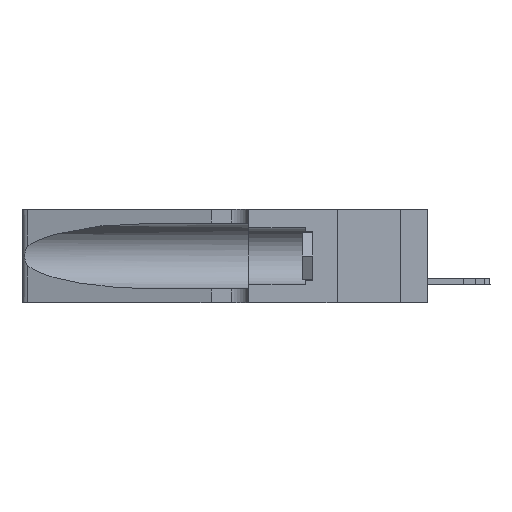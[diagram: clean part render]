
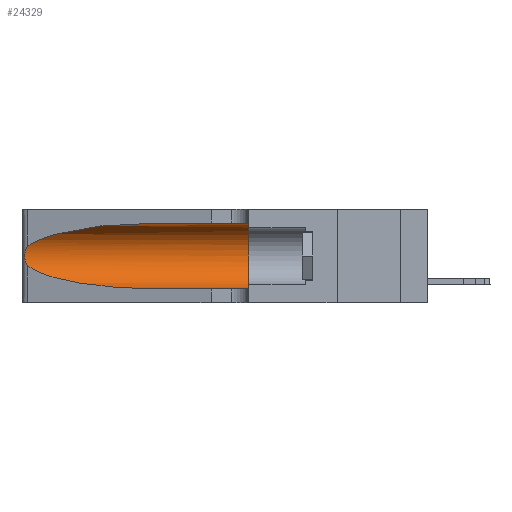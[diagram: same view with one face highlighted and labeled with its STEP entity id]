
A CAD part, left-side view. The second image highlights one B-rep face of the part: STEP entity #24329.
In plain terms, the highlighted cylindrical face has radius 3.308 mm (diameter 6.617 mm), a partial arc.
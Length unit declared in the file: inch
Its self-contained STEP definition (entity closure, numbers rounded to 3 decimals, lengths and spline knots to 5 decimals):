
#185 = VERTEX_POINT ( 'NONE', #25249 ) ;
#747 = ORIENTED_EDGE ( 'NONE', *, *, #14140, .T. ) ;
#1238 = CARTESIAN_POINT ( 'NONE',  ( 0.25487, 1.22718, 0.14631 ) ) ;
#2721 = CARTESIAN_POINT ( 'NONE',  ( 0.1305, 0.35, 0.31525 ) ) ;
#3000 = EDGE_CURVE ( 'NONE', #185, #18550, #15480, .T. ) ;
#3093 = CARTESIAN_POINT ( 'NONE',  ( 0.2373, 1.15595, 0.08982 ) ) ;
#3687 = EDGE_CURVE ( 'NONE', #185, #5527, #24208, .T. ) ;
#4220 = VERTEX_POINT ( 'NONE', #15285 ) ;
#4230 = CARTESIAN_POINT ( 'NONE',  ( 0.25487, 1.22718, 0.22369 ) ) ;
#4458 = CARTESIAN_POINT ( 'NONE',  ( 0.18966, 0.96281, 0.05475 ) ) ;
#4460 = CARTESIAN_POINT ( 'NONE',  ( 0.18966, 0.96281, 0.31525 ) ) ;
#4699 = ORIENTED_EDGE ( 'NONE', *, *, #13871, .T. ) ;
#5527 = VERTEX_POINT ( 'NONE', #9774 ) ;
#6185 = CARTESIAN_POINT ( 'NONE',  ( 0.25854, 1.2359, 0.20912 ) ) ;
#6305 = ORIENTED_EDGE ( 'NONE', *, *, #18896, .F. ) ;
#6319 = CARTESIAN_POINT ( 'NONE',  ( 0.1305, 0.72297, 0.31525 ) ) ;
#7128 = CARTESIAN_POINT ( 'NONE',  ( 0.25856, 1.23593, 0.16098 ) ) ;
#7228 = CARTESIAN_POINT ( 'NONE',  ( 0.25555, 1.22993, 0.14849 ) ) ;
#7884 = VECTOR ( 'NONE', #17106, 39.37008 ) ;
#8335 = CARTESIAN_POINT ( 'NONE',  ( 0.26075, 1.23896, 0.19203 ) ) ;
#8352 = AXIS2_PLACEMENT_3D ( 'NONE', #9111, #23697, #17482 ) ;
#8457 = CARTESIAN_POINT ( 'NONE',  ( 0.1305, 1.61858, 0.185 ) ) ;
#9111 = CARTESIAN_POINT ( 'NONE',  ( 0.1305, 0.35, 0.185 ) ) ;
#9644 = FACE_OUTER_BOUND ( 'NONE', #22752, .T. ) ;
#9720 = DIRECTION ( 'NONE',  ( 0., -1., 0. ) ) ;
#9774 = CARTESIAN_POINT ( 'NONE',  ( 0.25487, 1.22718, 0.22369 ) ) ;
#10078 = ORIENTED_EDGE ( 'NONE', *, *, #15621, .T. ) ;
#10710 =( BOUNDED_CURVE ( )  B_SPLINE_CURVE ( 3, ( #12504, #3093, #4458, #14472 ),
 .UNSPECIFIED., .F., .T. ) 
 B_SPLINE_CURVE_WITH_KNOTS ( ( 4, 4 ),
 ( 3.44316, 4.71239 ),
 .UNSPECIFIED. ) 
 CURVE ( )  GEOMETRIC_REPRESENTATION_ITEM ( )  RATIONAL_B_SPLINE_CURVE ( ( 1., 0.87, 0.87, 1. ) ) 
 REPRESENTATION_ITEM ( '' )  );
#11122 = AXIS2_PLACEMENT_3D ( 'NONE', #8457, #24713, #12396 ) ;
#12005 = CARTESIAN_POINT ( 'NONE',  ( 0.1305, 1.61858, 0.05475 ) ) ;
#12299 = CIRCLE ( 'NONE', #8352, 0.13025 ) ;
#12396 = DIRECTION ( 'NONE',  ( 0., 0., -1. ) ) ;
#12504 = CARTESIAN_POINT ( 'NONE',  ( 0.25487, 1.22718, 0.14631 ) ) ;
#13797 = VERTEX_POINT ( 'NONE', #20514 ) ;
#13871 = EDGE_CURVE ( 'NONE', #24351, #13797, #10710, .T. ) ;
#14140 = EDGE_CURVE ( 'NONE', #5527, #24351, #18557, .T. ) ;
#14472 = CARTESIAN_POINT ( 'NONE',  ( 0.1305, 0.72297, 0.05475 ) ) ;
#14692 = CYLINDRICAL_SURFACE ( 'NONE', #11122, 0.13025 ) ;
#15026 = CARTESIAN_POINT ( 'NONE',  ( 0.25789, 1.23486, 0.15765 ) ) ;
#15285 = CARTESIAN_POINT ( 'NONE',  ( 0.1305, 0.35, 0.05475 ) ) ;
#15480 = LINE ( 'NONE', #24943, #7884 ) ;
#15621 = EDGE_CURVE ( 'NONE', #13797, #4220, #15828, .T. ) ;
#15828 = LINE ( 'NONE', #12005, #22567 ) ;
#16533 = CARTESIAN_POINT ( 'NONE',  ( 0.2373, 1.15595, 0.28018 ) ) ;
#17106 = DIRECTION ( 'NONE',  ( 0., -1., 0. ) ) ;
#17187 = CARTESIAN_POINT ( 'NONE',  ( 0.26017, 1.23833, 0.17102 ) ) ;
#17482 = DIRECTION ( 'NONE',  ( 0., 0., 1. ) ) ;
#18550 = VERTEX_POINT ( 'NONE', #2721 ) ;
#18557 = B_SPLINE_CURVE_WITH_KNOTS ( 'NONE', 3,
 ( #4230, #22617, #24765, #20546, #6185, #20468, #8335, #18648, #17187, #7128, #15026, #23482, #7228, #1238 ),
 .UNSPECIFIED., .F., .F.,
 ( 4, 2, 2, 2, 2, 2, 4 ),
 ( 0., 0.00027, 0.00053, 0.00107, 0.0016, 0.00187, 0.00214 ),
 .UNSPECIFIED. ) ;
#18648 = CARTESIAN_POINT ( 'NONE',  ( 0.26075, 1.23896, 0.178 ) ) ;
#18896 = EDGE_CURVE ( 'NONE', #18550, #4220, #12299, .T. ) ;
#20468 = CARTESIAN_POINT ( 'NONE',  ( 0.26018, 1.23835, 0.19895 ) ) ;
#20514 = CARTESIAN_POINT ( 'NONE',  ( 0.1305, 0.72297, 0.05475 ) ) ;
#20546 = CARTESIAN_POINT ( 'NONE',  ( 0.25787, 1.23484, 0.2124 ) ) ;
#22567 = VECTOR ( 'NONE', #9720, 39.37008 ) ;
#22617 = CARTESIAN_POINT ( 'NONE',  ( 0.25555, 1.22994, 0.2215 ) ) ;
#22674 = CARTESIAN_POINT ( 'NONE',  ( 0.25487, 1.22718, 0.22369 ) ) ;
#22752 = EDGE_LOOP ( 'NONE', ( #23174, #747, #4699, #10078, #6305, #22986 ) ) ;
#22986 = ORIENTED_EDGE ( 'NONE', *, *, #3000, .F. ) ;
#23174 = ORIENTED_EDGE ( 'NONE', *, *, #3687, .T. ) ;
#23482 = CARTESIAN_POINT ( 'NONE',  ( 0.25639, 1.23186, 0.15144 ) ) ;
#23697 = DIRECTION ( 'NONE',  ( 0., 1., 0. ) ) ;
#24208 =( BOUNDED_CURVE ( )  B_SPLINE_CURVE ( 3, ( #6319, #4460, #16533, #22674 ),
 .UNSPECIFIED., .F., .T. ) 
 B_SPLINE_CURVE_WITH_KNOTS ( ( 4, 4 ),
 ( 1.5708, 2.84003 ),
 .UNSPECIFIED. ) 
 CURVE ( )  GEOMETRIC_REPRESENTATION_ITEM ( )  RATIONAL_B_SPLINE_CURVE ( ( 1., 0.87, 0.87, 1. ) ) 
 REPRESENTATION_ITEM ( '' )  );
#24329 = ADVANCED_FACE ( 'NONE', ( #9644 ), #14692, .F. ) ;
#24351 = VERTEX_POINT ( 'NONE', #24797 ) ;
#24713 = DIRECTION ( 'NONE',  ( 0., -1., 0. ) ) ;
#24765 = CARTESIAN_POINT ( 'NONE',  ( 0.25639, 1.23184, 0.21858 ) ) ;
#24797 = CARTESIAN_POINT ( 'NONE',  ( 0.25487, 1.22718, 0.14631 ) ) ;
#24943 = CARTESIAN_POINT ( 'NONE',  ( 0.1305, 1.61858, 0.31525 ) ) ;
#25249 = CARTESIAN_POINT ( 'NONE',  ( 0.1305, 0.72297, 0.31525 ) ) ;
